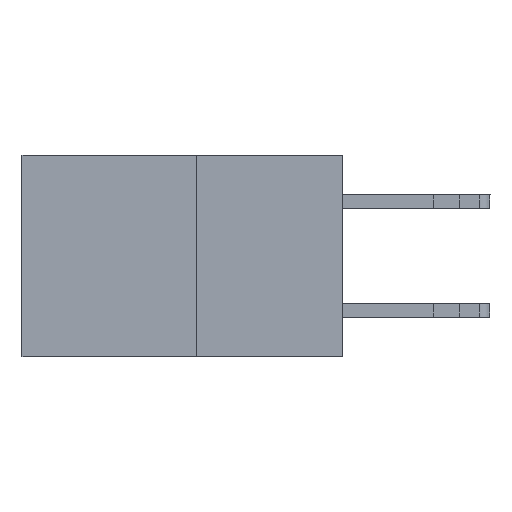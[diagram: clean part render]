
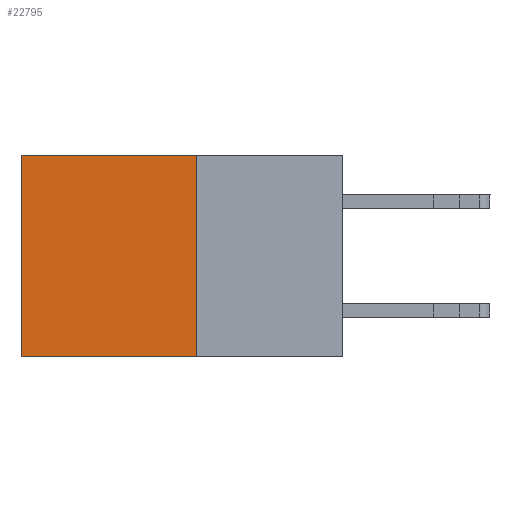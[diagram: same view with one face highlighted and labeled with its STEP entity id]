
A CAD part, left-side view. The second image highlights one B-rep face of the part: STEP entity #22795.
In plain terms, the highlighted planar face has unit normal (-1, 0, 0).
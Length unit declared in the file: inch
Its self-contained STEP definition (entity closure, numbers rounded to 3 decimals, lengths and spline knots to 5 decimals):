
#756 = AXIS2_PLACEMENT_3D ( 'NONE', #18009, #19505, #23599 ) ;
#938 = LINE ( 'NONE', #23234, #8407 ) ;
#1070 = FACE_OUTER_BOUND ( 'NONE', #12012, .T. ) ;
#2792 = PLANE ( 'NONE',  #756 ) ;
#3709 = ORIENTED_EDGE ( 'NONE', *, *, #10081, .F. ) ;
#4521 = ORIENTED_EDGE ( 'NONE', *, *, #24033, .T. ) ;
#6871 = EDGE_CURVE ( 'NONE', #12870, #14540, #20317, .T. ) ;
#8407 = VECTOR ( 'NONE', #8489, 39.37008 ) ;
#8489 = DIRECTION ( 'NONE',  ( 0., 1., 0. ) ) ;
#8687 = CARTESIAN_POINT ( 'NONE',  ( 0.277, 0.27, 0. ) ) ;
#9073 = CARTESIAN_POINT ( 'NONE',  ( 0.277, 0.27, -0.37 ) ) ;
#10081 = EDGE_CURVE ( 'NONE', #20114, #17508, #938, .T. ) ;
#11116 = ORIENTED_EDGE ( 'NONE', *, *, #6871, .T. ) ;
#11818 = LINE ( 'NONE', #23227, #12854 ) ;
#12012 = EDGE_LOOP ( 'NONE', ( #4521, #3709, #18021, #11116 ) ) ;
#12854 = VECTOR ( 'NONE', #17867, 39.37008 ) ;
#12870 = VERTEX_POINT ( 'NONE', #20117 ) ;
#14540 = VERTEX_POINT ( 'NONE', #19304 ) ;
#16927 = VECTOR ( 'NONE', #17483, 39.37008 ) ;
#17483 = DIRECTION ( 'NONE',  ( 0., 0., -1. ) ) ;
#17508 = VERTEX_POINT ( 'NONE', #17576 ) ;
#17576 = CARTESIAN_POINT ( 'NONE',  ( 0.277, 0.59, -0.37 ) ) ;
#17867 = DIRECTION ( 'NONE',  ( 0., 0., -1. ) ) ;
#17931 = EDGE_CURVE ( 'NONE', #12870, #20114, #11818, .T. ) ;
#18009 = CARTESIAN_POINT ( 'NONE',  ( 0.277, 0.27, -0.37 ) ) ;
#18021 = ORIENTED_EDGE ( 'NONE', *, *, #17931, .F. ) ;
#19304 = CARTESIAN_POINT ( 'NONE',  ( 0.277, 0.59, 0. ) ) ;
#19464 = CARTESIAN_POINT ( 'NONE',  ( 0.277, 0.59, -0.37 ) ) ;
#19505 = DIRECTION ( 'NONE',  ( 1., 0., 0. ) ) ;
#20114 = VERTEX_POINT ( 'NONE', #9073 ) ;
#20117 = CARTESIAN_POINT ( 'NONE',  ( 0.277, 0.27, 0. ) ) ;
#20317 = LINE ( 'NONE', #8687, #23777 ) ;
#21092 = LINE ( 'NONE', #19464, #16927 ) ;
#22795 = ADVANCED_FACE ( 'NONE', ( #1070 ), #2792, .F. ) ;
#23227 = CARTESIAN_POINT ( 'NONE',  ( 0.277, 0.27, -0.37 ) ) ;
#23234 = CARTESIAN_POINT ( 'NONE',  ( 0.277, 0.27, -0.37 ) ) ;
#23599 = DIRECTION ( 'NONE',  ( 0., 0., -1. ) ) ;
#23672 = DIRECTION ( 'NONE',  ( 0., 1., 0. ) ) ;
#23777 = VECTOR ( 'NONE', #23672, 39.37008 ) ;
#24033 = EDGE_CURVE ( 'NONE', #14540, #17508, #21092, .T. ) ;
